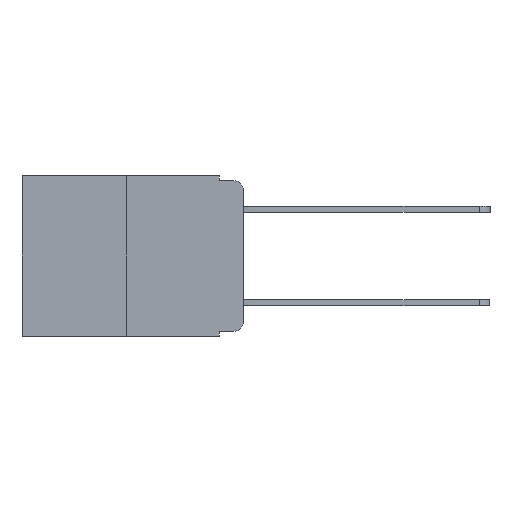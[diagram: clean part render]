
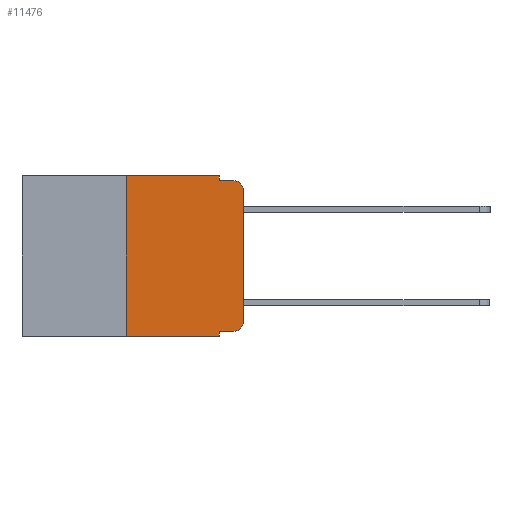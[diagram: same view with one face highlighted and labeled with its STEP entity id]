
A CAD part, left-side view. The second image highlights one B-rep face of the part: STEP entity #11476.
In plain terms, the highlighted planar face has unit normal (-1, 0, 0).
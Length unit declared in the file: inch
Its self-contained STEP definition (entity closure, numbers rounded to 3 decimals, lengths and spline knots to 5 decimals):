
#84 = ORIENTED_EDGE ( 'NONE', *, *, #3597, .T. ) ;
#130 = ORIENTED_EDGE ( 'NONE', *, *, #9993, .F. ) ;
#153 = LINE ( 'NONE', #5132, #16371 ) ;
#359 = AXIS2_PLACEMENT_3D ( 'NONE', #7097, #17718, #8702 ) ;
#858 = VERTEX_POINT ( 'NONE', #10418 ) ;
#1122 = ORIENTED_EDGE ( 'NONE', *, *, #12048, .T. ) ;
#1283 = ORIENTED_EDGE ( 'NONE', *, *, #8961, .F. ) ;
#1412 = EDGE_CURVE ( 'NONE', #858, #1723, #11434, .T. ) ;
#1435 = LINE ( 'NONE', #12716, #5246 ) ;
#1444 = ORIENTED_EDGE ( 'NONE', *, *, #4683, .F. ) ;
#1642 = ORIENTED_EDGE ( 'NONE', *, *, #8170, .T. ) ;
#1723 = VERTEX_POINT ( 'NONE', #18756 ) ;
#2032 = ORIENTED_EDGE ( 'NONE', *, *, #6796, .F. ) ;
#2233 = VECTOR ( 'NONE', #17738, 39.37008 ) ;
#2331 = ORIENTED_EDGE ( 'NONE', *, *, #6960, .F. ) ;
#2422 = VERTEX_POINT ( 'NONE', #3752 ) ;
#2568 = FACE_OUTER_BOUND ( 'NONE', #18443, .T. ) ;
#3166 = ORIENTED_EDGE ( 'NONE', *, *, #11029, .T. ) ;
#3597 = EDGE_CURVE ( 'NONE', #2422, #858, #1435, .T. ) ;
#3752 = CARTESIAN_POINT ( 'NONE',  ( 0., 0.051, -0.333 ) ) ;
#3775 = CARTESIAN_POINT ( 'NONE',  ( 0., 0.473, 0. ) ) ;
#4266 = CARTESIAN_POINT ( 'NONE',  ( 0., 0.051, -0.01 ) ) ;
#4683 = EDGE_CURVE ( 'NONE', #2422, #14088, #10609, .T. ) ;
#4894 = CARTESIAN_POINT ( 'NONE',  ( 0., 0., 0. ) ) ;
#5050 = DIRECTION ( 'NONE',  ( 0., 0., 1. ) ) ;
#5066 = VERTEX_POINT ( 'NONE', #8318 ) ;
#5132 = CARTESIAN_POINT ( 'NONE',  ( 0., 0.473, -0.343 ) ) ;
#5246 = VECTOR ( 'NONE', #10514, 39.37008 ) ;
#5848 = VECTOR ( 'NONE', #16158, 39.37008 ) ;
#6496 = DIRECTION ( 'NONE',  ( 0., 0., 1. ) ) ;
#6547 = DIRECTION ( 'NONE',  ( -1., 0., 0. ) ) ;
#6793 = CARTESIAN_POINT ( 'NONE',  ( 0., 0.02, -0.01 ) ) ;
#6796 = EDGE_CURVE ( 'NONE', #5066, #9604, #12949, .T. ) ;
#6960 = EDGE_CURVE ( 'NONE', #9604, #16465, #17545, .T. ) ;
#7097 = CARTESIAN_POINT ( 'NONE',  ( 0., 0.02, -0.03 ) ) ;
#7682 = VERTEX_POINT ( 'NONE', #6793 ) ;
#8170 = EDGE_CURVE ( 'NONE', #5066, #14088, #153, .T. ) ;
#8185 = CARTESIAN_POINT ( 'NONE',  ( 0., 0.25, 0. ) ) ;
#8255 = DIRECTION ( 'NONE',  ( 0., 0., -1. ) ) ;
#8272 = CARTESIAN_POINT ( 'NONE',  ( 0., 0.473, 0. ) ) ;
#8318 = CARTESIAN_POINT ( 'NONE',  ( 0., 0.25, -0.343 ) ) ;
#8554 = VECTOR ( 'NONE', #6496, 39.37008 ) ;
#8629 = CARTESIAN_POINT ( 'NONE',  ( 0., 0.25, 0. ) ) ;
#8702 = DIRECTION ( 'NONE',  ( 0., 0., -1. ) ) ;
#8961 = EDGE_CURVE ( 'NONE', #16465, #11820, #14254, .T. ) ;
#9078 = CARTESIAN_POINT ( 'NONE',  ( 0., 0.051, 0. ) ) ;
#9604 = VERTEX_POINT ( 'NONE', #8629 ) ;
#9803 = CARTESIAN_POINT ( 'NONE',  ( 0., 0.02, -0.313 ) ) ;
#9833 = DIRECTION ( 'NONE',  ( 0., 0., -1. ) ) ;
#9852 = CARTESIAN_POINT ( 'NONE',  ( 0., 0.051, -0.343 ) ) ;
#9993 = EDGE_CURVE ( 'NONE', #11820, #7682, #19688, .T. ) ;
#10301 = CARTESIAN_POINT ( 'NONE',  ( 0., 0.051, 0. ) ) ;
#10418 = CARTESIAN_POINT ( 'NONE',  ( 0., 0.02, -0.333 ) ) ;
#10514 = DIRECTION ( 'NONE',  ( 0., -1., 0. ) ) ;
#10609 = LINE ( 'NONE', #13988, #14171 ) ;
#11029 = EDGE_CURVE ( 'NONE', #16278, #7682, #11979, .T. ) ;
#11434 = CIRCLE ( 'NONE', #16755, 0.02 ) ;
#11476 = ADVANCED_FACE ( 'NONE', ( #2568 ), #17328, .F. ) ;
#11820 = VERTEX_POINT ( 'NONE', #4266 ) ;
#11841 = VECTOR ( 'NONE', #15712, 39.37008 ) ;
#11979 = CIRCLE ( 'NONE', #359, 0.02 ) ;
#12048 = EDGE_CURVE ( 'NONE', #1723, #16278, #16622, .T. ) ;
#12716 = CARTESIAN_POINT ( 'NONE',  ( 0., 0.051, -0.333 ) ) ;
#12949 = LINE ( 'NONE', #8185, #15944 ) ;
#13778 = AXIS2_PLACEMENT_3D ( 'NONE', #8272, #14356, #9833 ) ;
#13988 = CARTESIAN_POINT ( 'NONE',  ( 0., 0.051, 0. ) ) ;
#14088 = VERTEX_POINT ( 'NONE', #9852 ) ;
#14171 = VECTOR ( 'NONE', #19929, 39.37008 ) ;
#14238 = CARTESIAN_POINT ( 'NONE',  ( 0., 0.051, -0.01 ) ) ;
#14254 = LINE ( 'NONE', #10301, #2233 ) ;
#14356 = DIRECTION ( 'NONE',  ( 1., 0., 0. ) ) ;
#15712 = DIRECTION ( 'NONE',  ( 0., -1., 0. ) ) ;
#15944 = VECTOR ( 'NONE', #5050, 39.37008 ) ;
#16047 = ORIENTED_EDGE ( 'NONE', *, *, #1412, .T. ) ;
#16158 = DIRECTION ( 'NONE',  ( 0., -1., 0. ) ) ;
#16278 = VERTEX_POINT ( 'NONE', #19531 ) ;
#16371 = VECTOR ( 'NONE', #18842, 39.37008 ) ;
#16465 = VERTEX_POINT ( 'NONE', #9078 ) ;
#16622 = LINE ( 'NONE', #4894, #8554 ) ;
#16755 = AXIS2_PLACEMENT_3D ( 'NONE', #9803, #6547, #8255 ) ;
#17328 = PLANE ( 'NONE',  #13778 ) ;
#17545 = LINE ( 'NONE', #3775, #5848 ) ;
#17718 = DIRECTION ( 'NONE',  ( -1., 0., 0. ) ) ;
#17738 = DIRECTION ( 'NONE',  ( 0., 0., -1. ) ) ;
#18443 = EDGE_LOOP ( 'NONE', ( #1122, #3166, #130, #1283, #2331, #2032, #1642, #1444, #84, #16047 ) ) ;
#18756 = CARTESIAN_POINT ( 'NONE',  ( 0., 0., -0.313 ) ) ;
#18842 = DIRECTION ( 'NONE',  ( 0., -1., 0. ) ) ;
#19531 = CARTESIAN_POINT ( 'NONE',  ( 0., 0., -0.03 ) ) ;
#19688 = LINE ( 'NONE', #14238, #11841 ) ;
#19929 = DIRECTION ( 'NONE',  ( 0., 0., -1. ) ) ;
